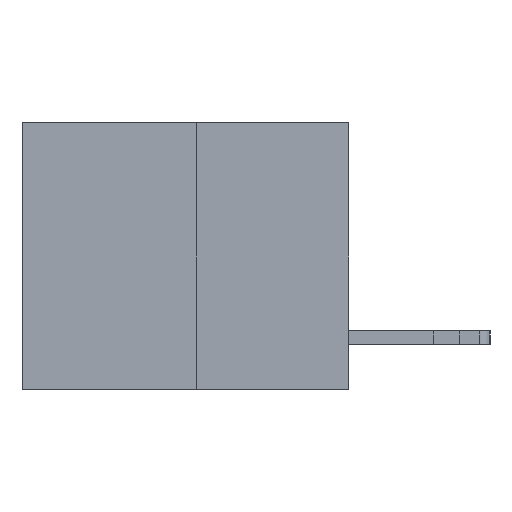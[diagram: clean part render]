
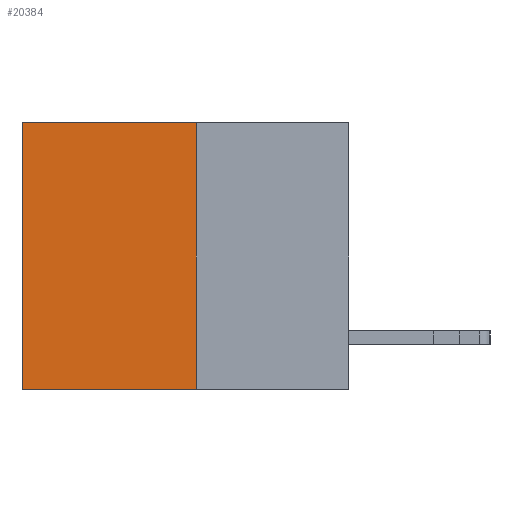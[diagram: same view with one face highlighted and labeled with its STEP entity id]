
A CAD part, left-side view. The second image highlights one B-rep face of the part: STEP entity #20384.
In plain terms, the highlighted planar face has unit normal (-1, 0, 0).
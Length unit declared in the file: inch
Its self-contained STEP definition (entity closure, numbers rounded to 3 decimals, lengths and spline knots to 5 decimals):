
#349 = DIRECTION ( 'NONE',  ( 0., 1., 0. ) ) ;
#1334 = VECTOR ( 'NONE', #349, 39.37008 ) ;
#1605 = EDGE_CURVE ( 'NONE', #10765, #18719, #22673, .T. ) ;
#3887 = LINE ( 'NONE', #17930, #20050 ) ;
#4156 = ORIENTED_EDGE ( 'NONE', *, *, #5561, .T. ) ;
#4417 = ORIENTED_EDGE ( 'NONE', *, *, #11847, .T. ) ;
#5013 = ORIENTED_EDGE ( 'NONE', *, *, #15998, .F. ) ;
#5561 = EDGE_CURVE ( 'NONE', #28081, #18719, #3887, .T. ) ;
#7002 = DIRECTION ( 'NONE',  ( 0., 0., -1. ) ) ;
#7364 = DIRECTION ( 'NONE',  ( 0., 0., -1. ) ) ;
#10765 = VERTEX_POINT ( 'NONE', #16270 ) ;
#11068 = LINE ( 'NONE', #25376, #23143 ) ;
#11691 = CARTESIAN_POINT ( 'NONE',  ( 0.3165, 0.6, -0.49 ) ) ;
#11847 = EDGE_CURVE ( 'NONE', #24867, #28081, #11068, .T. ) ;
#12538 = PLANE ( 'NONE',  #28257 ) ;
#14420 = DIRECTION ( 'NONE',  ( 0., 1., 0. ) ) ;
#14777 = DIRECTION ( 'NONE',  ( 0., 0., -1. ) ) ;
#14972 = CARTESIAN_POINT ( 'NONE',  ( 0.3165, 0.28, -0.49 ) ) ;
#15998 = EDGE_CURVE ( 'NONE', #24867, #10765, #16931, .T. ) ;
#16270 = CARTESIAN_POINT ( 'NONE',  ( 0.3165, 0.28, -0.49 ) ) ;
#16931 = LINE ( 'NONE', #27009, #27256 ) ;
#17930 = CARTESIAN_POINT ( 'NONE',  ( 0.3165, 0.6, -0.49 ) ) ;
#18719 = VERTEX_POINT ( 'NONE', #11691 ) ;
#19876 = CARTESIAN_POINT ( 'NONE',  ( 0.3165, 0.28, -0.49 ) ) ;
#20050 = VECTOR ( 'NONE', #7364, 39.37008 ) ;
#20384 = ADVANCED_FACE ( 'NONE', ( #22273 ), #12538, .F. ) ;
#21597 = DIRECTION ( 'NONE',  ( 1., 0., 0. ) ) ;
#21893 = CARTESIAN_POINT ( 'NONE',  ( 0.3165, 0.28, 0. ) ) ;
#22273 = FACE_OUTER_BOUND ( 'NONE', #24788, .T. ) ;
#22673 = LINE ( 'NONE', #19876, #1334 ) ;
#23143 = VECTOR ( 'NONE', #14420, 39.37008 ) ;
#24788 = EDGE_LOOP ( 'NONE', ( #4156, #26120, #5013, #4417 ) ) ;
#24867 = VERTEX_POINT ( 'NONE', #21893 ) ;
#25376 = CARTESIAN_POINT ( 'NONE',  ( 0.3165, 0.28, 0. ) ) ;
#26120 = ORIENTED_EDGE ( 'NONE', *, *, #1605, .F. ) ;
#27009 = CARTESIAN_POINT ( 'NONE',  ( 0.3165, 0.28, -0.49 ) ) ;
#27256 = VECTOR ( 'NONE', #7002, 39.37008 ) ;
#28081 = VERTEX_POINT ( 'NONE', #28224 ) ;
#28224 = CARTESIAN_POINT ( 'NONE',  ( 0.3165, 0.6, 0. ) ) ;
#28257 = AXIS2_PLACEMENT_3D ( 'NONE', #14972, #21597, #14777 ) ;
